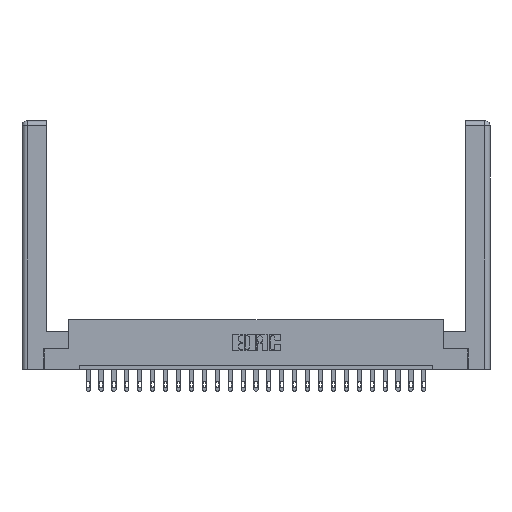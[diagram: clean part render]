
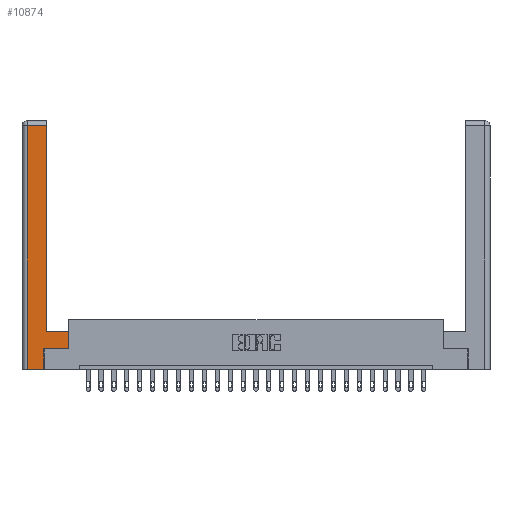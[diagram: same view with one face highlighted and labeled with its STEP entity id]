
A CAD part, top view. The second image highlights one B-rep face of the part: STEP entity #10874.
In plain terms, the highlighted planar face has unit normal (0, 0, 1).
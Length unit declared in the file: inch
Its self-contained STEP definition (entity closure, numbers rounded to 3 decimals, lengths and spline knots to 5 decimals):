
#87 = VERTEX_POINT ( 'NONE', #18849 ) ;
#261 = CARTESIAN_POINT ( 'NONE',  ( 0.565, 0.245, 0. ) ) ;
#270 = FACE_OUTER_BOUND ( 'NONE', #7675, .T. ) ;
#858 = CARTESIAN_POINT ( 'NONE',  ( 0.265, 0., 0. ) ) ;
#873 = EDGE_CURVE ( 'NONE', #1060, #8088, #1167, .T. ) ;
#1060 = VERTEX_POINT ( 'NONE', #858 ) ;
#1106 = CARTESIAN_POINT ( 'NONE',  ( 0.565, 0.45, 0. ) ) ;
#1167 = LINE ( 'NONE', #12885, #20771 ) ;
#1193 = EDGE_CURVE ( 'NONE', #87, #21911, #9734, .T. ) ;
#1604 = CARTESIAN_POINT ( 'NONE',  ( 0.0615, 2.94, 0. ) ) ;
#2541 = CARTESIAN_POINT ( 'NONE',  ( 0.295, 2.94, 0. ) ) ;
#2942 = LINE ( 'NONE', #9612, #7665 ) ;
#3183 = CARTESIAN_POINT ( 'NONE',  ( 0., 0., 0. ) ) ;
#4147 = CARTESIAN_POINT ( 'NONE',  ( 0.295, 3., 0. ) ) ;
#4447 = EDGE_CURVE ( 'NONE', #13723, #11804, #10043, .T. ) ;
#4798 = VECTOR ( 'NONE', #5594, 39.37008 ) ;
#5017 = PLANE ( 'NONE',  #5332 ) ;
#5080 = LINE ( 'NONE', #13046, #4798 ) ;
#5332 = AXIS2_PLACEMENT_3D ( 'NONE', #3183, #14189, #22203 ) ;
#5580 = LINE ( 'NONE', #23814, #19218 ) ;
#5594 = DIRECTION ( 'NONE',  ( -1., 0., 0. ) ) ;
#5822 = DIRECTION ( 'NONE',  ( 1., 0., 0. ) ) ;
#5900 = VERTEX_POINT ( 'NONE', #19060 ) ;
#6351 = CARTESIAN_POINT ( 'NONE',  ( 0.295, 0.45, 0. ) ) ;
#7328 = DIRECTION ( 'NONE',  ( -1., 0., 0. ) ) ;
#7665 = VECTOR ( 'NONE', #13489, 39.37008 ) ;
#7675 = EDGE_LOOP ( 'NONE', ( #9987, #17891, #16349, #18810, #15633, #20890, #12198, #10036 ) ) ;
#7729 = CARTESIAN_POINT ( 'NONE',  ( 0.265, 0.245, 0. ) ) ;
#8088 = VERTEX_POINT ( 'NONE', #7729 ) ;
#8654 = DIRECTION ( 'NONE',  ( 0., 1., 0. ) ) ;
#9612 = CARTESIAN_POINT ( 'NONE',  ( 0.265, 0., 0. ) ) ;
#9734 = LINE ( 'NONE', #1106, #13001 ) ;
#9987 = ORIENTED_EDGE ( 'NONE', *, *, #4447, .T. ) ;
#10036 = ORIENTED_EDGE ( 'NONE', *, *, #21025, .T. ) ;
#10043 = LINE ( 'NONE', #4147, #22158 ) ;
#10396 = VECTOR ( 'NONE', #7328, 39.37008 ) ;
#10874 = ADVANCED_FACE ( 'NONE', ( #270 ), #5017, .F. ) ;
#11305 = EDGE_CURVE ( 'NONE', #5900, #1060, #2942, .T. ) ;
#11415 = EDGE_CURVE ( 'NONE', #21357, #5900, #5580, .T. ) ;
#11804 = VERTEX_POINT ( 'NONE', #2541 ) ;
#12060 = CARTESIAN_POINT ( 'NONE',  ( 0.565, 0.45, 0. ) ) ;
#12198 = ORIENTED_EDGE ( 'NONE', *, *, #1193, .T. ) ;
#12413 = DIRECTION ( 'NONE',  ( 0., -1., 0. ) ) ;
#12885 = CARTESIAN_POINT ( 'NONE',  ( 0.265, 0.245, 0. ) ) ;
#13001 = VECTOR ( 'NONE', #8654, 39.37008 ) ;
#13046 = CARTESIAN_POINT ( 'NONE',  ( 0.295, 0.45, 0. ) ) ;
#13489 = DIRECTION ( 'NONE',  ( 1., 0., 0. ) ) ;
#13669 = DIRECTION ( 'NONE',  ( 0., 1., 0. ) ) ;
#13723 = VERTEX_POINT ( 'NONE', #6351 ) ;
#14189 = DIRECTION ( 'NONE',  ( 0., 0., -1. ) ) ;
#15633 = ORIENTED_EDGE ( 'NONE', *, *, #873, .T. ) ;
#15937 = VECTOR ( 'NONE', #5822, 39.37008 ) ;
#16349 = ORIENTED_EDGE ( 'NONE', *, *, #11415, .T. ) ;
#17891 = ORIENTED_EDGE ( 'NONE', *, *, #21141, .T. ) ;
#18518 = DIRECTION ( 'NONE',  ( 0., 1., 0. ) ) ;
#18810 = ORIENTED_EDGE ( 'NONE', *, *, #11305, .T. ) ;
#18849 = CARTESIAN_POINT ( 'NONE',  ( 0.565, 0.245, 0. ) ) ;
#19060 = CARTESIAN_POINT ( 'NONE',  ( 0.0615, 0., 0. ) ) ;
#19218 = VECTOR ( 'NONE', #12413, 39.37008 ) ;
#19844 = CARTESIAN_POINT ( 'NONE',  ( 0.0615, 2.94, 0. ) ) ;
#20771 = VECTOR ( 'NONE', #18518, 39.37008 ) ;
#20890 = ORIENTED_EDGE ( 'NONE', *, *, #23031, .T. ) ;
#21025 = EDGE_CURVE ( 'NONE', #21911, #13723, #5080, .T. ) ;
#21058 = LINE ( 'NONE', #261, #15937 ) ;
#21141 = EDGE_CURVE ( 'NONE', #11804, #21357, #23168, .T. ) ;
#21357 = VERTEX_POINT ( 'NONE', #19844 ) ;
#21911 = VERTEX_POINT ( 'NONE', #12060 ) ;
#22158 = VECTOR ( 'NONE', #13669, 39.37008 ) ;
#22203 = DIRECTION ( 'NONE',  ( -1., 0., 0. ) ) ;
#23031 = EDGE_CURVE ( 'NONE', #8088, #87, #21058, .T. ) ;
#23168 = LINE ( 'NONE', #1604, #10396 ) ;
#23814 = CARTESIAN_POINT ( 'NONE',  ( 0.0615, 0., 0. ) ) ;
